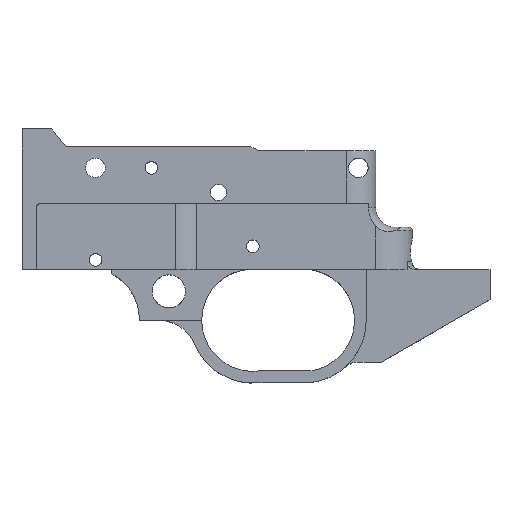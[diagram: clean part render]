
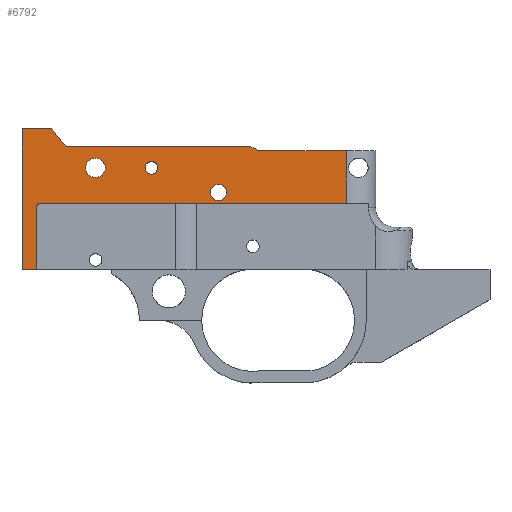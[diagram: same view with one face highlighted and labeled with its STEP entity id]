
A CAD part, top view. The second image highlights one B-rep face of the part: STEP entity #6792.
In plain terms, the highlighted planar face has unit normal (0, 0, 1).
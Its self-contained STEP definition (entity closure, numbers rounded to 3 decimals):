
#178 = CARTESIAN_POINT ( 'NONE',  ( 1.26, 30.5, 30.327 ) ) ;
#297 = EDGE_CURVE ( 'NONE', #8492, #3857, #2952, .T. ) ;
#326 = VERTEX_POINT ( 'NONE', #3049 ) ;
#408 = DIRECTION ( 'NONE',  ( 1., 0., 0. ) ) ;
#456 = FACE_OUTER_BOUND ( 'NONE', #4838, .T. ) ;
#488 = CARTESIAN_POINT ( 'NONE',  ( -89.44, 0., 30.327 ) ) ;
#597 = DIRECTION ( 'NONE',  ( 0., 0., 1. ) ) ;
#773 = VECTOR ( 'NONE', #7006, 1000. ) ;
#836 = ORIENTED_EDGE ( 'NONE', *, *, #4098, .T. ) ;
#955 = LINE ( 'NONE', #5454, #6217 ) ;
#1043 = DIRECTION ( 'NONE',  ( 1., 0., 0. ) ) ;
#1046 = CIRCLE ( 'NONE', #6552, 1.625 ) ;
#1088 = CARTESIAN_POINT ( 'NONE',  ( -81.84, 36.08, 30.327 ) ) ;
#1141 = CARTESIAN_POINT ( 'NONE',  ( -28.74, 30.5, 30.327 ) ) ;
#1185 = VECTOR ( 'NONE', #6641, 1000. ) ;
#1327 = EDGE_LOOP ( 'NONE', ( #1948, #3260 ) ) ;
#1371 = EDGE_CURVE ( 'NONE', #3524, #3749, #2423, .T. ) ;
#1392 = CARTESIAN_POINT ( 'NONE',  ( -70.61, 26.1, 30.327 ) ) ;
#1525 = AXIS2_PLACEMENT_3D ( 'NONE', #1629, #6252, #2293 ) ;
#1629 = CARTESIAN_POINT ( 'NONE',  ( -84.69, 16., 30.327 ) ) ;
#1648 = EDGE_CURVE ( 'NONE', #326, #4802, #6025, .T. ) ;
#1880 = CARTESIAN_POINT ( 'NONE',  ( -57.885, 26.1, 30.327 ) ) ;
#1948 = ORIENTED_EDGE ( 'NONE', *, *, #6122, .F. ) ;
#2018 = AXIS2_PLACEMENT_3D ( 'NONE', #1392, #5991, #2032 ) ;
#2023 = EDGE_CURVE ( 'NONE', #6734, #3924, #4165, .T. ) ;
#2032 = DIRECTION ( 'NONE',  ( 1., 0., 0. ) ) ;
#2037 = ORIENTED_EDGE ( 'NONE', *, *, #5639, .F. ) ;
#2102 = EDGE_CURVE ( 'NONE', #7115, #7256, #3754, .T. ) ;
#2197 = FACE_BOUND ( 'NONE', #2711, .T. ) ;
#2203 = EDGE_CURVE ( 'NONE', #5282, #5046, #3325, .T. ) ;
#2205 = CARTESIAN_POINT ( 'NONE',  ( -78.14, 31.5, 30.327 ) ) ;
#2258 = VERTEX_POINT ( 'NONE', #2449 ) ;
#2293 = DIRECTION ( 'NONE',  ( -1., 0., 0. ) ) ;
#2306 = AXIS2_PLACEMENT_3D ( 'NONE', #7032, #3076, #7711 ) ;
#2312 = DIRECTION ( 'NONE',  ( 1., 0., 0. ) ) ;
#2423 = CIRCLE ( 'NONE', #3443, 2.5 ) ;
#2449 = CARTESIAN_POINT ( 'NONE',  ( -54.635, 26.1, 30.327 ) ) ;
#2591 = EDGE_CURVE ( 'NONE', #5046, #3857, #6329, .T. ) ;
#2711 = EDGE_LOOP ( 'NONE', ( #6479, #2037 ) ) ;
#2744 = VECTOR ( 'NONE', #8353, 1000. ) ;
#2762 = DIRECTION ( 'NONE',  ( 1., 0., 0. ) ) ;
#2786 = CARTESIAN_POINT ( 'NONE',  ( -56.26, 26.1, 30.327 ) ) ;
#2884 = ORIENTED_EDGE ( 'NONE', *, *, #1648, .F. ) ;
#2952 = LINE ( 'NONE', #7022, #2744 ) ;
#2968 = CARTESIAN_POINT ( 'NONE',  ( -70.61, 26.1, 30.327 ) ) ;
#3048 = DIRECTION ( 'NONE',  ( 0., -1., 0. ) ) ;
#3049 = CARTESIAN_POINT ( 'NONE',  ( -41.14, 19.8, 30.327 ) ) ;
#3058 = CARTESIAN_POINT ( 'NONE',  ( -85.69, 17., 30.327 ) ) ;
#3076 = DIRECTION ( 'NONE',  ( 0., 0., 1. ) ) ;
#3260 = ORIENTED_EDGE ( 'NONE', *, *, #3927, .F. ) ;
#3277 = AXIS2_PLACEMENT_3D ( 'NONE', #8319, #4349, #408 ) ;
#3325 = LINE ( 'NONE', #7670, #8402 ) ;
#3410 = CARTESIAN_POINT ( 'NONE',  ( -6.24, 30.5, 30.327 ) ) ;
#3443 = AXIS2_PLACEMENT_3D ( 'NONE', #2968, #6925, #2312 ) ;
#3444 = DIRECTION ( 'NONE',  ( 1., 0., 0. ) ) ;
#3469 = CARTESIAN_POINT ( 'NONE',  ( -81.84, 36.08, 30.327 ) ) ;
#3524 = VERTEX_POINT ( 'NONE', #4941 ) ;
#3633 = EDGE_CURVE ( 'NONE', #4802, #326, #4449, .T. ) ;
#3639 = ORIENTED_EDGE ( 'NONE', *, *, #4681, .F. ) ;
#3640 = CIRCLE ( 'NONE', #6291, 1.625 ) ;
#3749 = VERTEX_POINT ( 'NONE', #4496 ) ;
#3754 = LINE ( 'NONE', #3469, #5296 ) ;
#3857 = VERTEX_POINT ( 'NONE', #5901 ) ;
#3924 = VERTEX_POINT ( 'NONE', #3410 ) ;
#3927 = EDGE_CURVE ( 'NONE', #4893, #2258, #1046, .T. ) ;
#3947 = VECTOR ( 'NONE', #6741, 1000. ) ;
#4021 = AXIS2_PLACEMENT_3D ( 'NONE', #7174, #8502, #4539 ) ;
#4026 = VERTEX_POINT ( 'NONE', #7493 ) ;
#4098 = EDGE_CURVE ( 'NONE', #8492, #4026, #7020, .T. ) ;
#4165 = LINE ( 'NONE', #178, #3947 ) ;
#4292 = DIRECTION ( 'NONE',  ( -0.628, 0.778, 0. ) ) ;
#4349 = DIRECTION ( 'NONE',  ( 0., 0., 1. ) ) ;
#4373 = LINE ( 'NONE', #4724, #5915 ) ;
#4449 = CIRCLE ( 'NONE', #2306, 2.1 ) ;
#4496 = CARTESIAN_POINT ( 'NONE',  ( -73.11, 26.1, 30.327 ) ) ;
#4539 = DIRECTION ( 'NONE',  ( -1., 0., 0. ) ) ;
#4542 = CARTESIAN_POINT ( 'NONE',  ( -56.26, 26.1, 30.327 ) ) ;
#4569 = CIRCLE ( 'NONE', #2018, 2.5 ) ;
#4681 = EDGE_CURVE ( 'NONE', #7115, #5651, #6244, .T. ) ;
#4724 = CARTESIAN_POINT ( 'NONE',  ( -89.44, 36.08, 30.327 ) ) ;
#4740 = EDGE_CURVE ( 'NONE', #6274, #4026, #6028, .T. ) ;
#4750 = CARTESIAN_POINT ( 'NONE',  ( -89.44, 0., 30.327 ) ) ;
#4802 = VERTEX_POINT ( 'NONE', #5715 ) ;
#4826 = ORIENTED_EDGE ( 'NONE', *, *, #7695, .T. ) ;
#4838 = EDGE_LOOP ( 'NONE', ( #7165, #4826, #6090, #7047, #3639, #8152, #5587, #5807, #6587, #7431, #836 ) ) ;
#4893 = VERTEX_POINT ( 'NONE', #1880 ) ;
#4941 = CARTESIAN_POINT ( 'NONE',  ( -68.11, 26.1, 30.327 ) ) ;
#5043 = EDGE_CURVE ( 'NONE', #5282, #7256, #4373, .T. ) ;
#5046 = VERTEX_POINT ( 'NONE', #4750 ) ;
#5112 = DIRECTION ( 'NONE',  ( 1., 0., 0. ) ) ;
#5215 = DIRECTION ( 'NONE',  ( 1., 0., 0. ) ) ;
#5282 = VERTEX_POINT ( 'NONE', #7677 ) ;
#5296 = VECTOR ( 'NONE', #4292, 1000. ) ;
#5336 = CARTESIAN_POINT ( 'NONE',  ( -30.74, 31.5, 30.327 ) ) ;
#5393 = ORIENTED_EDGE ( 'NONE', *, *, #3633, .F. ) ;
#5454 = CARTESIAN_POINT ( 'NONE',  ( -6.24, 31.5, 30.327 ) ) ;
#5587 = ORIENTED_EDGE ( 'NONE', *, *, #5043, .F. ) ;
#5639 = EDGE_CURVE ( 'NONE', #3749, #3524, #4569, .T. ) ;
#5648 = CARTESIAN_POINT ( 'NONE',  ( -89.44, 31.5, 30.327 ) ) ;
#5651 = VERTEX_POINT ( 'NONE', #5336 ) ;
#5715 = CARTESIAN_POINT ( 'NONE',  ( -36.94, 19.8, 30.327 ) ) ;
#5807 = ORIENTED_EDGE ( 'NONE', *, *, #2203, .T. ) ;
#5840 = PLANE ( 'NONE',  #4021 ) ;
#5901 = CARTESIAN_POINT ( 'NONE',  ( -85.69, 0., 30.327 ) ) ;
#5915 = VECTOR ( 'NONE', #2762, 1000. ) ;
#5968 = CARTESIAN_POINT ( 'NONE',  ( -30.74, 31.5, 30.327 ) ) ;
#5991 = DIRECTION ( 'NONE',  ( 0., 0., 1. ) ) ;
#6025 = CIRCLE ( 'NONE', #3277, 2.1 ) ;
#6028 = LINE ( 'NONE', #3058, #773 ) ;
#6083 = EDGE_LOOP ( 'NONE', ( #5393, #2884 ) ) ;
#6090 = ORIENTED_EDGE ( 'NONE', *, *, #2023, .F. ) ;
#6115 = DIRECTION ( 'NONE',  ( 0., 1., 0. ) ) ;
#6122 = EDGE_CURVE ( 'NONE', #2258, #4893, #3640, .T. ) ;
#6217 = VECTOR ( 'NONE', #6115, 1000. ) ;
#6244 = LINE ( 'NONE', #5648, #8003 ) ;
#6252 = DIRECTION ( 'NONE',  ( 0., 0., -1. ) ) ;
#6274 = VERTEX_POINT ( 'NONE', #7912 ) ;
#6291 = AXIS2_PLACEMENT_3D ( 'NONE', #4542, #597, #5215 ) ;
#6300 = EDGE_CURVE ( 'NONE', #5651, #6734, #6438, .T. ) ;
#6329 = LINE ( 'NONE', #488, #6530 ) ;
#6438 = LINE ( 'NONE', #5968, #1185 ) ;
#6479 = ORIENTED_EDGE ( 'NONE', *, *, #1371, .F. ) ;
#6530 = VECTOR ( 'NONE', #5112, 1000. ) ;
#6552 = AXIS2_PLACEMENT_3D ( 'NONE', #2786, #7402, #3444 ) ;
#6587 = ORIENTED_EDGE ( 'NONE', *, *, #2591, .T. ) ;
#6641 = DIRECTION ( 'NONE',  ( 0.894, -0.447, 0. ) ) ;
#6734 = VERTEX_POINT ( 'NONE', #1141 ) ;
#6741 = DIRECTION ( 'NONE',  ( 1., 0., 0. ) ) ;
#6792 = ADVANCED_FACE ( 'NONE', ( #7257, #7469, #2197, #456 ), #5840, .F. ) ;
#6925 = DIRECTION ( 'NONE',  ( 0., 0., 1. ) ) ;
#7006 = DIRECTION ( 'NONE',  ( -1., 0., 0. ) ) ;
#7020 = CIRCLE ( 'NONE', #1525, 1. ) ;
#7022 = CARTESIAN_POINT ( 'NONE',  ( -85.69, 0., 30.327 ) ) ;
#7032 = CARTESIAN_POINT ( 'NONE',  ( -39.04, 19.8, 30.327 ) ) ;
#7047 = ORIENTED_EDGE ( 'NONE', *, *, #6300, .F. ) ;
#7115 = VERTEX_POINT ( 'NONE', #2205 ) ;
#7129 = CARTESIAN_POINT ( 'NONE',  ( -85.69, 16., 30.327 ) ) ;
#7165 = ORIENTED_EDGE ( 'NONE', *, *, #4740, .F. ) ;
#7174 = CARTESIAN_POINT ( 'NONE',  ( -89.44, 31.5, 30.327 ) ) ;
#7256 = VERTEX_POINT ( 'NONE', #1088 ) ;
#7257 = FACE_BOUND ( 'NONE', #6083, .T. ) ;
#7402 = DIRECTION ( 'NONE',  ( 0., 0., 1. ) ) ;
#7431 = ORIENTED_EDGE ( 'NONE', *, *, #297, .F. ) ;
#7469 = FACE_BOUND ( 'NONE', #1327, .T. ) ;
#7493 = CARTESIAN_POINT ( 'NONE',  ( -84.69, 17., 30.327 ) ) ;
#7670 = CARTESIAN_POINT ( 'NONE',  ( -89.44, 31.5, 30.327 ) ) ;
#7677 = CARTESIAN_POINT ( 'NONE',  ( -89.44, 36.08, 30.327 ) ) ;
#7695 = EDGE_CURVE ( 'NONE', #6274, #3924, #955, .T. ) ;
#7711 = DIRECTION ( 'NONE',  ( 1., 0., 0. ) ) ;
#7912 = CARTESIAN_POINT ( 'NONE',  ( -6.24, 17., 30.327 ) ) ;
#8003 = VECTOR ( 'NONE', #1043, 1000. ) ;
#8152 = ORIENTED_EDGE ( 'NONE', *, *, #2102, .T. ) ;
#8319 = CARTESIAN_POINT ( 'NONE',  ( -39.04, 19.8, 30.327 ) ) ;
#8353 = DIRECTION ( 'NONE',  ( 0., -1., 0. ) ) ;
#8402 = VECTOR ( 'NONE', #3048, 1000. ) ;
#8492 = VERTEX_POINT ( 'NONE', #7129 ) ;
#8502 = DIRECTION ( 'NONE',  ( 0., 0., -1. ) ) ;
